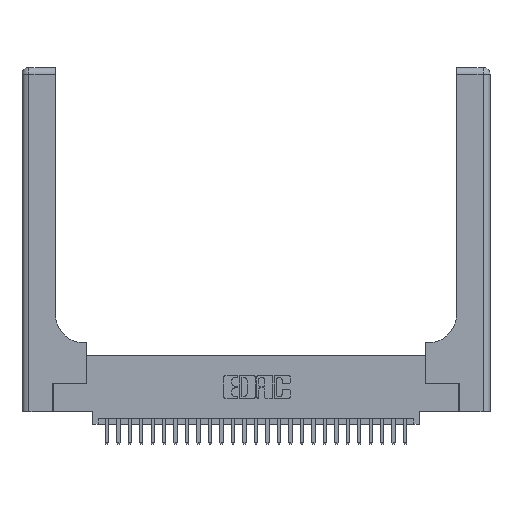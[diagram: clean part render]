
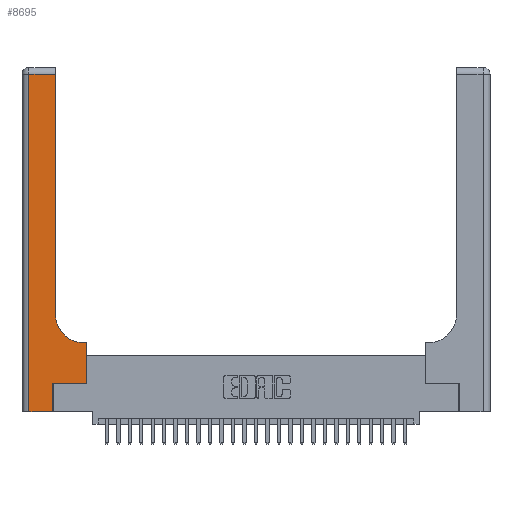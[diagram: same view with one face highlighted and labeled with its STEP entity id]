
A CAD part, top view. The second image highlights one B-rep face of the part: STEP entity #8695.
In plain terms, the highlighted planar face has unit normal (0, 0, 1).
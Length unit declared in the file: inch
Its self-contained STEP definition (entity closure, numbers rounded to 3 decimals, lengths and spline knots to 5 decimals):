
#98 = LINE ( 'NONE', #17044, #28471 ) ;
#135 = CARTESIAN_POINT ( 'NONE',  ( 0.06, 0., 0.37 ) ) ;
#716 = PLANE ( 'NONE',  #23704 ) ;
#1086 = CARTESIAN_POINT ( 'NONE',  ( 0.269, 0., 0.37 ) ) ;
#1100 = CARTESIAN_POINT ( 'NONE',  ( 0.269, 0., 0.37 ) ) ;
#1167 = DIRECTION ( 'NONE',  ( 0., 1., 0. ) ) ;
#1961 = ORIENTED_EDGE ( 'NONE', *, *, #3367, .T. ) ;
#2534 = VECTOR ( 'NONE', #12543, 39.37008 ) ;
#2922 = ORIENTED_EDGE ( 'NONE', *, *, #3241, .T. ) ;
#2941 = CIRCLE ( 'NONE', #26332, 0.25 ) ;
#3241 = EDGE_CURVE ( 'NONE', #9245, #17613, #15958, .T. ) ;
#3325 = DIRECTION ( 'NONE',  ( 0., 1., 0. ) ) ;
#3367 = EDGE_CURVE ( 'NONE', #8207, #9245, #17371, .T. ) ;
#5090 = ORIENTED_EDGE ( 'NONE', *, *, #19557, .T. ) ;
#5626 = DIRECTION ( 'NONE',  ( 1., 0., 0. ) ) ;
#7166 = CARTESIAN_POINT ( 'NONE',  ( 0., 3., 0.37 ) ) ;
#7452 = CARTESIAN_POINT ( 'NONE',  ( 0.5585, 0.25, 0.37 ) ) ;
#7593 = ORIENTED_EDGE ( 'NONE', *, *, #23779, .T. ) ;
#7733 = VECTOR ( 'NONE', #24779, 39.37008 ) ;
#8207 = VERTEX_POINT ( 'NONE', #26325 ) ;
#8491 = CARTESIAN_POINT ( 'NONE',  ( 0.269, 0.25, 0.37 ) ) ;
#8509 = VERTEX_POINT ( 'NONE', #22638 ) ;
#8695 = ADVANCED_FACE ( 'NONE', ( #14721 ), #716, .F. ) ;
#9245 = VERTEX_POINT ( 'NONE', #11057 ) ;
#9587 = CARTESIAN_POINT ( 'NONE',  ( 0.5415, 0.6, 0.37 ) ) ;
#10431 = EDGE_CURVE ( 'NONE', #17613, #25569, #98, .T. ) ;
#10679 = VECTOR ( 'NONE', #20411, 39.37008 ) ;
#11057 = CARTESIAN_POINT ( 'NONE',  ( 0.06, 2.94, 0.37 ) ) ;
#11533 = CARTESIAN_POINT ( 'NONE',  ( 0.2915, 0.6, 0.37 ) ) ;
#11630 = DIRECTION ( 'NONE',  ( 1., 0., 0. ) ) ;
#11655 = DIRECTION ( 'NONE',  ( -1., 0., 0. ) ) ;
#12267 = DIRECTION ( 'NONE',  ( 0., 0., -1. ) ) ;
#12543 = DIRECTION ( 'NONE',  ( 0., -1., 0. ) ) ;
#12837 = VERTEX_POINT ( 'NONE', #9587 ) ;
#13373 = VERTEX_POINT ( 'NONE', #8491 ) ;
#13483 = CARTESIAN_POINT ( 'NONE',  ( 0.5585, 0.25, 0.37 ) ) ;
#14028 = ORIENTED_EDGE ( 'NONE', *, *, #23856, .T. ) ;
#14298 = EDGE_CURVE ( 'NONE', #12837, #20057, #2941, .T. ) ;
#14496 = DIRECTION ( 'NONE',  ( 1., 0., 0. ) ) ;
#14721 = FACE_OUTER_BOUND ( 'NONE', #19746, .T. ) ;
#14991 = LINE ( 'NONE', #13483, #7733 ) ;
#15198 = ORIENTED_EDGE ( 'NONE', *, *, #14298, .T. ) ;
#15958 = LINE ( 'NONE', #25766, #2534 ) ;
#16532 = CARTESIAN_POINT ( 'NONE',  ( 0., 2.94, 0.37 ) ) ;
#16537 = LINE ( 'NONE', #11533, #10679 ) ;
#17044 = CARTESIAN_POINT ( 'NONE',  ( 0., 0., 0.37 ) ) ;
#17371 = LINE ( 'NONE', #16532, #23276 ) ;
#17613 = VERTEX_POINT ( 'NONE', #135 ) ;
#17678 = ORIENTED_EDGE ( 'NONE', *, *, #17915, .T. ) ;
#17905 = VERTEX_POINT ( 'NONE', #7452 ) ;
#17915 = EDGE_CURVE ( 'NONE', #25569, #13373, #18894, .T. ) ;
#18385 = DIRECTION ( 'NONE',  ( 0., 0., -1. ) ) ;
#18732 = CARTESIAN_POINT ( 'NONE',  ( 0.2915, 3., 0.37 ) ) ;
#18894 = LINE ( 'NONE', #1100, #22727 ) ;
#19557 = EDGE_CURVE ( 'NONE', #17905, #8509, #14991, .T. ) ;
#19591 = ORIENTED_EDGE ( 'NONE', *, *, #27701, .T. ) ;
#19746 = EDGE_LOOP ( 'NONE', ( #19591, #1961, #2922, #21786, #17678, #7593, #5090, #14028, #15198 ) ) ;
#20057 = VERTEX_POINT ( 'NONE', #26369 ) ;
#20158 = VECTOR ( 'NONE', #1167, 39.37008 ) ;
#20311 = CARTESIAN_POINT ( 'NONE',  ( 0.269, 0.25, 0.37 ) ) ;
#20411 = DIRECTION ( 'NONE',  ( -1., 0., 0. ) ) ;
#20981 = DIRECTION ( 'NONE',  ( -1., 0., 0. ) ) ;
#21786 = ORIENTED_EDGE ( 'NONE', *, *, #10431, .T. ) ;
#22065 = LINE ( 'NONE', #20311, #22429 ) ;
#22429 = VECTOR ( 'NONE', #11630, 39.37008 ) ;
#22638 = CARTESIAN_POINT ( 'NONE',  ( 0.5585, 0.6, 0.37 ) ) ;
#22727 = VECTOR ( 'NONE', #3325, 39.37008 ) ;
#23276 = VECTOR ( 'NONE', #20981, 39.37008 ) ;
#23704 = AXIS2_PLACEMENT_3D ( 'NONE', #7166, #18385, #11655 ) ;
#23779 = EDGE_CURVE ( 'NONE', #13373, #17905, #22065, .T. ) ;
#23856 = EDGE_CURVE ( 'NONE', #8509, #12837, #16537, .T. ) ;
#24779 = DIRECTION ( 'NONE',  ( 0., 1., 0. ) ) ;
#25332 = LINE ( 'NONE', #18732, #20158 ) ;
#25569 = VERTEX_POINT ( 'NONE', #1086 ) ;
#25692 = CARTESIAN_POINT ( 'NONE',  ( 0.5415, 0.85, 0.37 ) ) ;
#25766 = CARTESIAN_POINT ( 'NONE',  ( 0.06, 3., 0.37 ) ) ;
#26325 = CARTESIAN_POINT ( 'NONE',  ( 0.2915, 2.94, 0.37 ) ) ;
#26332 = AXIS2_PLACEMENT_3D ( 'NONE', #25692, #12267, #14496 ) ;
#26369 = CARTESIAN_POINT ( 'NONE',  ( 0.2915, 0.85, 0.37 ) ) ;
#27701 = EDGE_CURVE ( 'NONE', #20057, #8207, #25332, .T. ) ;
#28471 = VECTOR ( 'NONE', #5626, 39.37008 ) ;
